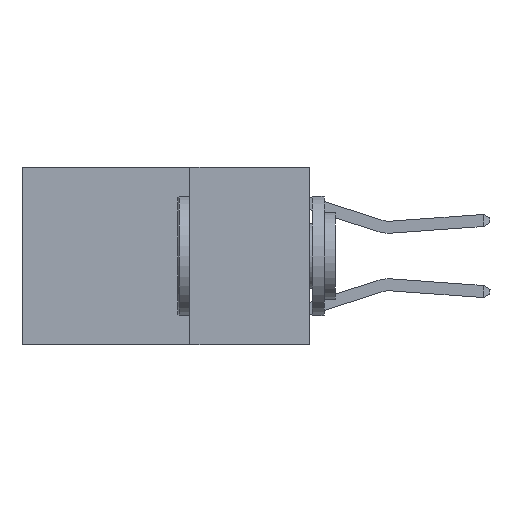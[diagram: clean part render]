
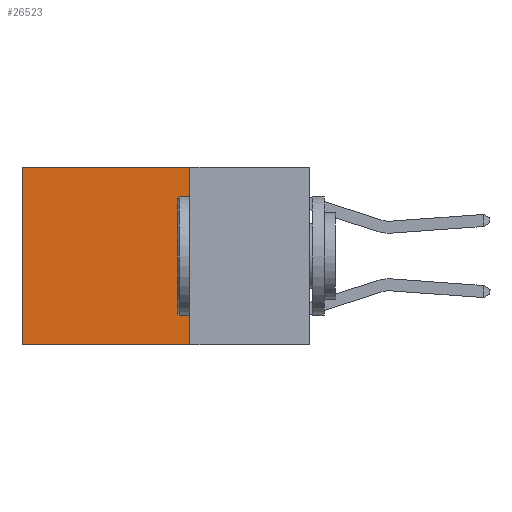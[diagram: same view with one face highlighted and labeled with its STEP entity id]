
A CAD part, left-side view. The second image highlights one B-rep face of the part: STEP entity #26523.
In plain terms, the highlighted planar face has unit normal (-1, 0, 0).
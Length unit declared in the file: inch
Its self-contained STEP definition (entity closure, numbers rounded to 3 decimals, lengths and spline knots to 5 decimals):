
#190 = LINE ( 'NONE', #30708, #20591 ) ;
#222 = CARTESIAN_POINT ( 'NONE',  ( 0.2625, 0.25, -0.37 ) ) ;
#401 = EDGE_LOOP ( 'NONE', ( #14457, #29872, #21558, #12700 ) ) ;
#847 = CARTESIAN_POINT ( 'NONE',  ( 0.2625, 0.6, 0. ) ) ;
#4166 = CARTESIAN_POINT ( 'NONE',  ( 0.2625, 0.25, 0. ) ) ;
#4399 = DIRECTION ( 'NONE',  ( 0., 0., -1. ) ) ;
#5340 = DIRECTION ( 'NONE',  ( 0., 0., -1. ) ) ;
#6543 = CARTESIAN_POINT ( 'NONE',  ( 0.2625, 0.25, 0. ) ) ;
#7533 = CARTESIAN_POINT ( 'NONE',  ( 0.2625, 0.6, 0. ) ) ;
#7761 = VECTOR ( 'NONE', #5340, 39.37008 ) ;
#7916 = CARTESIAN_POINT ( 'NONE',  ( 0.2625, 0.25, 0. ) ) ;
#8990 = VERTEX_POINT ( 'NONE', #7916 ) ;
#9116 = DIRECTION ( 'NONE',  ( 0., 1., 0. ) ) ;
#9864 = AXIS2_PLACEMENT_3D ( 'NONE', #4166, #13936, #4399 ) ;
#11476 = VERTEX_POINT ( 'NONE', #22355 ) ;
#12470 = EDGE_CURVE ( 'NONE', #8990, #28230, #31338, .T. ) ;
#12647 = VECTOR ( 'NONE', #29863, 39.37008 ) ;
#12700 = ORIENTED_EDGE ( 'NONE', *, *, #12470, .T. ) ;
#12864 = VECTOR ( 'NONE', #9116, 39.37008 ) ;
#13064 = CARTESIAN_POINT ( 'NONE',  ( 0.2625, 0.25, -0.37 ) ) ;
#13936 = DIRECTION ( 'NONE',  ( 1., 0., 0. ) ) ;
#14457 = ORIENTED_EDGE ( 'NONE', *, *, #18731, .T. ) ;
#15750 = EDGE_CURVE ( 'NONE', #8990, #24544, #190, .T. ) ;
#16577 = FACE_OUTER_BOUND ( 'NONE', #401, .T. ) ;
#18731 = EDGE_CURVE ( 'NONE', #28230, #11476, #26668, .T. ) ;
#20591 = VECTOR ( 'NONE', #23340, 39.37008 ) ;
#21558 = ORIENTED_EDGE ( 'NONE', *, *, #15750, .F. ) ;
#22334 = LINE ( 'NONE', #13064, #12647 ) ;
#22355 = CARTESIAN_POINT ( 'NONE',  ( 0.2625, 0.6, -0.37 ) ) ;
#23340 = DIRECTION ( 'NONE',  ( 0., 0., -1. ) ) ;
#24544 = VERTEX_POINT ( 'NONE', #222 ) ;
#26523 = ADVANCED_FACE ( 'NONE', ( #16577 ), #31374, .F. ) ;
#26668 = LINE ( 'NONE', #7533, #7761 ) ;
#27607 = EDGE_CURVE ( 'NONE', #24544, #11476, #22334, .T. ) ;
#28230 = VERTEX_POINT ( 'NONE', #847 ) ;
#29863 = DIRECTION ( 'NONE',  ( 0., 1., 0. ) ) ;
#29872 = ORIENTED_EDGE ( 'NONE', *, *, #27607, .F. ) ;
#30708 = CARTESIAN_POINT ( 'NONE',  ( 0.2625, 0.25, 0. ) ) ;
#31338 = LINE ( 'NONE', #6543, #12864 ) ;
#31374 = PLANE ( 'NONE',  #9864 ) ;
